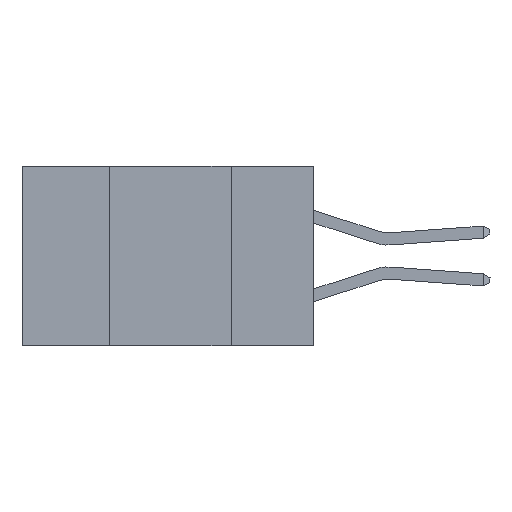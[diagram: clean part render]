
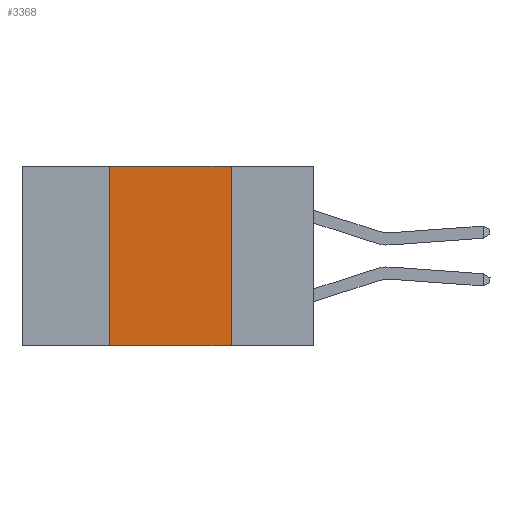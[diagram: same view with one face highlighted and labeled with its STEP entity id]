
A CAD part, left-side view. The second image highlights one B-rep face of the part: STEP entity #3368.
In plain terms, the highlighted planar face has unit normal (-1, 0, 0).
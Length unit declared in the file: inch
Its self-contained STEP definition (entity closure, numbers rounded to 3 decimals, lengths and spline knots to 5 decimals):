
#276 = VERTEX_POINT ( 'NONE', #16380 ) ;
#761 = CARTESIAN_POINT ( 'NONE',  ( 0., 0.42, 0. ) ) ;
#1640 = CARTESIAN_POINT ( 'NONE',  ( 0., 0.17, 0. ) ) ;
#1660 = EDGE_CURVE ( 'NONE', #14474, #276, #5765, .T. ) ;
#3368 = ADVANCED_FACE ( 'NONE', ( #15160 ), #16591, .F. ) ;
#3497 = CARTESIAN_POINT ( 'NONE',  ( 0., 0.6, 0. ) ) ;
#5303 = CARTESIAN_POINT ( 'NONE',  ( 0., 0.42, 0. ) ) ;
#5734 = CARTESIAN_POINT ( 'NONE',  ( 0., 0.6, 0. ) ) ;
#5749 = DIRECTION ( 'NONE',  ( 0., -1., 0. ) ) ;
#5765 = LINE ( 'NONE', #16960, #17166 ) ;
#5898 = EDGE_CURVE ( 'NONE', #14474, #7535, #18186, .T. ) ;
#6672 = EDGE_CURVE ( 'NONE', #7535, #11897, #7729, .T. ) ;
#6889 = DIRECTION ( 'NONE',  ( 0., 0., 1. ) ) ;
#7237 = VECTOR ( 'NONE', #8223, 39.37008 ) ;
#7302 = DIRECTION ( 'NONE',  ( 1., 0., 0. ) ) ;
#7535 = VERTEX_POINT ( 'NONE', #761 ) ;
#7729 = LINE ( 'NONE', #3497, #7237 ) ;
#8223 = DIRECTION ( 'NONE',  ( 0., -1., 0. ) ) ;
#8397 = DIRECTION ( 'NONE',  ( 0., 0., -1. ) ) ;
#8878 = ORIENTED_EDGE ( 'NONE', *, *, #6672, .F. ) ;
#10995 = ORIENTED_EDGE ( 'NONE', *, *, #5898, .F. ) ;
#11462 = ORIENTED_EDGE ( 'NONE', *, *, #13492, .F. ) ;
#11897 = VERTEX_POINT ( 'NONE', #1640 ) ;
#12500 = ORIENTED_EDGE ( 'NONE', *, *, #1660, .T. ) ;
#13492 = EDGE_CURVE ( 'NONE', #11897, #276, #17306, .T. ) ;
#13633 = CARTESIAN_POINT ( 'NONE',  ( 0., 0.42, -0.37 ) ) ;
#14000 = VECTOR ( 'NONE', #6889, 39.37008 ) ;
#14474 = VERTEX_POINT ( 'NONE', #13633 ) ;
#15160 = FACE_OUTER_BOUND ( 'NONE', #15958, .T. ) ;
#15958 = EDGE_LOOP ( 'NONE', ( #11462, #8878, #10995, #12500 ) ) ;
#16380 = CARTESIAN_POINT ( 'NONE',  ( 0., 0.17, -0.37 ) ) ;
#16591 = PLANE ( 'NONE',  #19414 ) ;
#16960 = CARTESIAN_POINT ( 'NONE',  ( 0., 0.6, -0.37 ) ) ;
#17166 = VECTOR ( 'NONE', #5749, 39.37008 ) ;
#17306 = LINE ( 'NONE', #19219, #17797 ) ;
#17797 = VECTOR ( 'NONE', #8397, 39.37008 ) ;
#18146 = DIRECTION ( 'NONE',  ( 0., 0., -1. ) ) ;
#18186 = LINE ( 'NONE', #5303, #14000 ) ;
#19219 = CARTESIAN_POINT ( 'NONE',  ( 0., 0.17, 0. ) ) ;
#19414 = AXIS2_PLACEMENT_3D ( 'NONE', #5734, #7302, #18146 ) ;
